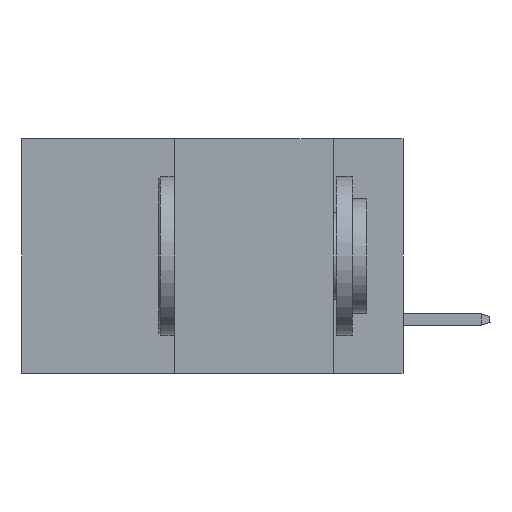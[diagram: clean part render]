
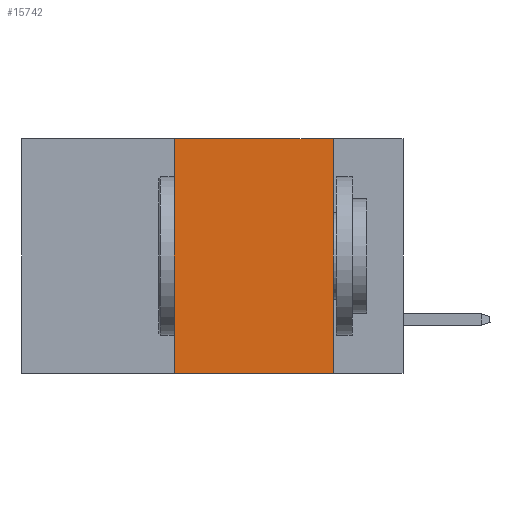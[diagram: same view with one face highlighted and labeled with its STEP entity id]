
A CAD part, left-side view. The second image highlights one B-rep face of the part: STEP entity #15742.
In plain terms, the highlighted planar face has unit normal (-1, 0, 0).
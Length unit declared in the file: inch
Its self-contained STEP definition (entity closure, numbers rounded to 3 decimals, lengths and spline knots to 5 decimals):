
#1644 = VERTEX_POINT ( 'NONE', #18743 ) ;
#1732 = DIRECTION ( 'NONE',  ( 1., 0., 0. ) ) ;
#2105 = CARTESIAN_POINT ( 'NONE',  ( 0., 0.6, -0.37 ) ) ;
#2628 = CARTESIAN_POINT ( 'NONE',  ( 0., 0.11, 0. ) ) ;
#3011 = EDGE_CURVE ( 'NONE', #1644, #19425, #20614, .T. ) ;
#3021 = VECTOR ( 'NONE', #8562, 39.37008 ) ;
#3219 = EDGE_LOOP ( 'NONE', ( #4341, #11976, #19927, #23701 ) ) ;
#3762 = EDGE_CURVE ( 'NONE', #4020, #11799, #4312, .T. ) ;
#4020 = VERTEX_POINT ( 'NONE', #5594 ) ;
#4312 = LINE ( 'NONE', #2105, #8434 ) ;
#4341 = ORIENTED_EDGE ( 'NONE', *, *, #21697, .F. ) ;
#5380 = CARTESIAN_POINT ( 'NONE',  ( 0., 0.36, 0. ) ) ;
#5594 = CARTESIAN_POINT ( 'NONE',  ( 0., 0.36, -0.37 ) ) ;
#7959 = DIRECTION ( 'NONE',  ( 0., -1., 0. ) ) ;
#8304 = CARTESIAN_POINT ( 'NONE',  ( 0., 0.6, 0. ) ) ;
#8434 = VECTOR ( 'NONE', #7959, 39.37008 ) ;
#8562 = DIRECTION ( 'NONE',  ( 0., 0., -1. ) ) ;
#11799 = VERTEX_POINT ( 'NONE', #17807 ) ;
#11954 = LINE ( 'NONE', #14266, #3021 ) ;
#11976 = ORIENTED_EDGE ( 'NONE', *, *, #3011, .F. ) ;
#12757 = EDGE_CURVE ( 'NONE', #4020, #1644, #25376, .T. ) ;
#13564 = FACE_OUTER_BOUND ( 'NONE', #3219, .T. ) ;
#14266 = CARTESIAN_POINT ( 'NONE',  ( 0., 0.11, 0. ) ) ;
#15742 = ADVANCED_FACE ( 'NONE', ( #13564 ), #21450, .F. ) ;
#16384 = AXIS2_PLACEMENT_3D ( 'NONE', #19472, #1732, #17566 ) ;
#17285 = VECTOR ( 'NONE', #25134, 39.37008 ) ;
#17532 = VECTOR ( 'NONE', #20351, 39.37008 ) ;
#17566 = DIRECTION ( 'NONE',  ( 0., 0., -1. ) ) ;
#17807 = CARTESIAN_POINT ( 'NONE',  ( 0., 0.11, -0.37 ) ) ;
#18743 = CARTESIAN_POINT ( 'NONE',  ( 0., 0.36, 0. ) ) ;
#19425 = VERTEX_POINT ( 'NONE', #2628 ) ;
#19472 = CARTESIAN_POINT ( 'NONE',  ( 0., 0.6, 0. ) ) ;
#19927 = ORIENTED_EDGE ( 'NONE', *, *, #12757, .F. ) ;
#20351 = DIRECTION ( 'NONE',  ( 0., -1., 0. ) ) ;
#20614 = LINE ( 'NONE', #8304, #17532 ) ;
#21450 = PLANE ( 'NONE',  #16384 ) ;
#21697 = EDGE_CURVE ( 'NONE', #19425, #11799, #11954, .T. ) ;
#23701 = ORIENTED_EDGE ( 'NONE', *, *, #3762, .T. ) ;
#25134 = DIRECTION ( 'NONE',  ( 0., 0., 1. ) ) ;
#25376 = LINE ( 'NONE', #5380, #17285 ) ;
